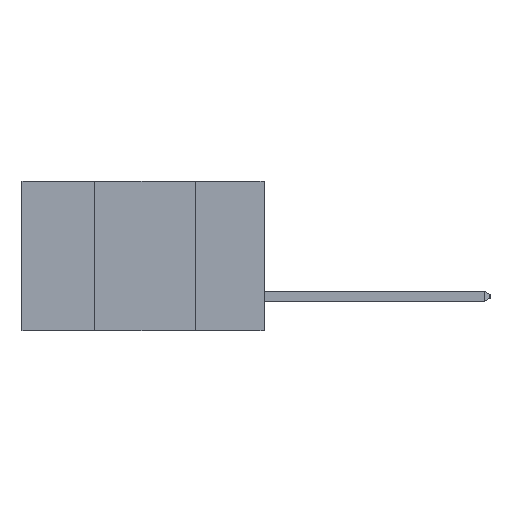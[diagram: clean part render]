
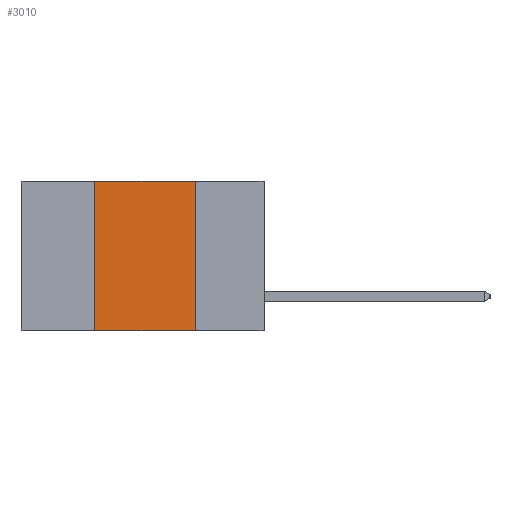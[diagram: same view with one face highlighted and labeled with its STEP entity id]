
A CAD part, left-side view. The second image highlights one B-rep face of the part: STEP entity #3010.
In plain terms, the highlighted planar face has unit normal (-1, 0, 0).
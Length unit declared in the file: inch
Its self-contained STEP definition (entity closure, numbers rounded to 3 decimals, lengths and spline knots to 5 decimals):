
#1126 = CARTESIAN_POINT ( 'NONE',  ( 0., 0.17, -0.37 ) ) ;
#1278 = LINE ( 'NONE', #15627, #14028 ) ;
#2236 = ORIENTED_EDGE ( 'NONE', *, *, #8757, .T. ) ;
#2485 = CARTESIAN_POINT ( 'NONE',  ( 0., 0.17, 0. ) ) ;
#3010 = ADVANCED_FACE ( 'NONE', ( #15574 ), #8034, .F. ) ;
#4113 = CARTESIAN_POINT ( 'NONE',  ( 0., 0.42, 0. ) ) ;
#4267 = ORIENTED_EDGE ( 'NONE', *, *, #11071, .F. ) ;
#4866 = VERTEX_POINT ( 'NONE', #2485 ) ;
#4951 = ORIENTED_EDGE ( 'NONE', *, *, #12913, .F. ) ;
#5678 = DIRECTION ( 'NONE',  ( 0., -1., 0. ) ) ;
#5706 = VERTEX_POINT ( 'NONE', #4113 ) ;
#5880 = ORIENTED_EDGE ( 'NONE', *, *, #9514, .F. ) ;
#7668 = LINE ( 'NONE', #15219, #13587 ) ;
#7963 = CARTESIAN_POINT ( 'NONE',  ( 0., 0.6, 0. ) ) ;
#8019 = VECTOR ( 'NONE', #5678, 39.37008 ) ;
#8034 = PLANE ( 'NONE',  #10049 ) ;
#8121 = DIRECTION ( 'NONE',  ( 0., 0., -1. ) ) ;
#8181 = DIRECTION ( 'NONE',  ( 1., 0., 0. ) ) ;
#8593 = DIRECTION ( 'NONE',  ( 0., 0., 1. ) ) ;
#8605 = VERTEX_POINT ( 'NONE', #11861 ) ;
#8757 = EDGE_CURVE ( 'NONE', #8605, #11920, #15382, .T. ) ;
#9514 = EDGE_CURVE ( 'NONE', #8605, #5706, #1278, .T. ) ;
#10049 = AXIS2_PLACEMENT_3D ( 'NONE', #7963, #8181, #8121 ) ;
#11071 = EDGE_CURVE ( 'NONE', #4866, #11920, #7668, .T. ) ;
#11130 = LINE ( 'NONE', #14011, #8019 ) ;
#11782 = VECTOR ( 'NONE', #15772, 39.37008 ) ;
#11861 = CARTESIAN_POINT ( 'NONE',  ( 0., 0.42, -0.37 ) ) ;
#11920 = VERTEX_POINT ( 'NONE', #1126 ) ;
#12913 = EDGE_CURVE ( 'NONE', #5706, #4866, #11130, .T. ) ;
#13377 = CARTESIAN_POINT ( 'NONE',  ( 0., 0.6, -0.37 ) ) ;
#13462 = EDGE_LOOP ( 'NONE', ( #4267, #4951, #5880, #2236 ) ) ;
#13587 = VECTOR ( 'NONE', #13994, 39.37008 ) ;
#13994 = DIRECTION ( 'NONE',  ( 0., 0., -1. ) ) ;
#14011 = CARTESIAN_POINT ( 'NONE',  ( 0., 0.6, 0. ) ) ;
#14028 = VECTOR ( 'NONE', #8593, 39.37008 ) ;
#15219 = CARTESIAN_POINT ( 'NONE',  ( 0., 0.17, 0. ) ) ;
#15382 = LINE ( 'NONE', #13377, #11782 ) ;
#15574 = FACE_OUTER_BOUND ( 'NONE', #13462, .T. ) ;
#15627 = CARTESIAN_POINT ( 'NONE',  ( 0., 0.42, 0. ) ) ;
#15772 = DIRECTION ( 'NONE',  ( 0., -1., 0. ) ) ;
